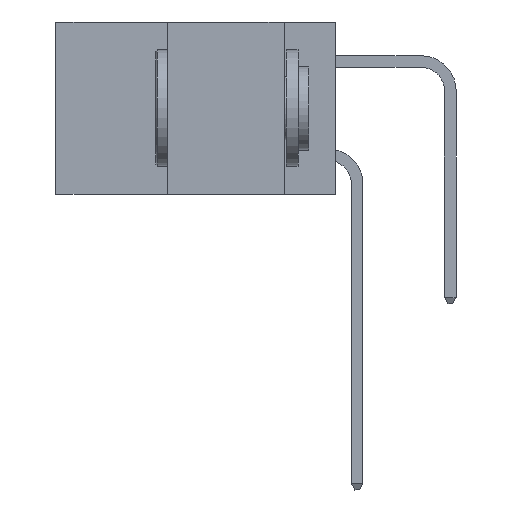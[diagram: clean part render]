
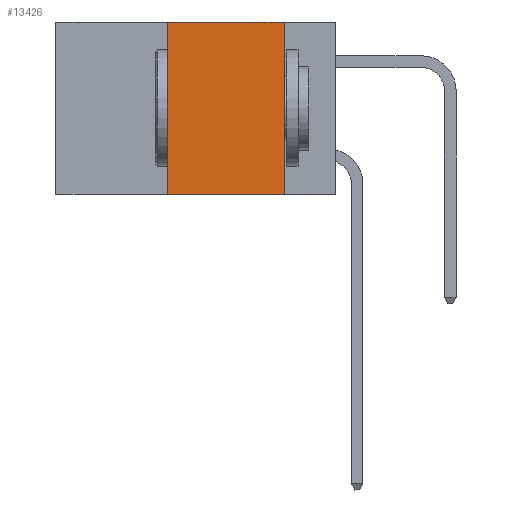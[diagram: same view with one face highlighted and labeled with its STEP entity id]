
A CAD part, left-side view. The second image highlights one B-rep face of the part: STEP entity #13426.
In plain terms, the highlighted planar face has unit normal (-1, 0, 0).
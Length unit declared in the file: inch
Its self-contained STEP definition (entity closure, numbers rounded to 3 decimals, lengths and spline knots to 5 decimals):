
#1444 = CARTESIAN_POINT ( 'NONE',  ( 0., 0.11, 0. ) ) ;
#1592 = VERTEX_POINT ( 'NONE', #6874 ) ;
#1670 = LINE ( 'NONE', #9726, #9550 ) ;
#1695 = DIRECTION ( 'NONE',  ( 0., 0., -1. ) ) ;
#2039 = LINE ( 'NONE', #3371, #7864 ) ;
#2083 = ORIENTED_EDGE ( 'NONE', *, *, #8110, .F. ) ;
#2244 = CARTESIAN_POINT ( 'NONE',  ( 0., 0.36, 0. ) ) ;
#2601 = CARTESIAN_POINT ( 'NONE',  ( 0., 0.6, 0. ) ) ;
#3084 = DIRECTION ( 'NONE',  ( 0., -1., 0. ) ) ;
#3119 = VECTOR ( 'NONE', #12470, 39.37008 ) ;
#3371 = CARTESIAN_POINT ( 'NONE',  ( 0., 0.6, -0.37 ) ) ;
#3650 = EDGE_CURVE ( 'NONE', #6396, #1592, #12769, .T. ) ;
#4830 = LINE ( 'NONE', #1444, #9013 ) ;
#4873 = DIRECTION ( 'NONE',  ( 0., 0., -1. ) ) ;
#5020 = AXIS2_PLACEMENT_3D ( 'NONE', #2601, #7124, #4873 ) ;
#5290 = EDGE_CURVE ( 'NONE', #6396, #11457, #2039, .T. ) ;
#5695 = ORIENTED_EDGE ( 'NONE', *, *, #8839, .F. ) ;
#5762 = CARTESIAN_POINT ( 'NONE',  ( 0., 0.36, -0.37 ) ) ;
#6326 = CARTESIAN_POINT ( 'NONE',  ( 0., 0.11, 0. ) ) ;
#6396 = VERTEX_POINT ( 'NONE', #5762 ) ;
#6810 = DIRECTION ( 'NONE',  ( 0., -1., 0. ) ) ;
#6874 = CARTESIAN_POINT ( 'NONE',  ( 0., 0.36, 0. ) ) ;
#6894 = ORIENTED_EDGE ( 'NONE', *, *, #3650, .F. ) ;
#7075 = PLANE ( 'NONE',  #5020 ) ;
#7124 = DIRECTION ( 'NONE',  ( 1., 0., 0. ) ) ;
#7228 = FACE_OUTER_BOUND ( 'NONE', #11441, .T. ) ;
#7864 = VECTOR ( 'NONE', #6810, 39.37008 ) ;
#8110 = EDGE_CURVE ( 'NONE', #1592, #8829, #1670, .T. ) ;
#8829 = VERTEX_POINT ( 'NONE', #6326 ) ;
#8839 = EDGE_CURVE ( 'NONE', #8829, #11457, #4830, .T. ) ;
#9013 = VECTOR ( 'NONE', #1695, 39.37008 ) ;
#9550 = VECTOR ( 'NONE', #3084, 39.37008 ) ;
#9726 = CARTESIAN_POINT ( 'NONE',  ( 0., 0.6, 0. ) ) ;
#11441 = EDGE_LOOP ( 'NONE', ( #5695, #2083, #6894, #13343 ) ) ;
#11457 = VERTEX_POINT ( 'NONE', #11888 ) ;
#11888 = CARTESIAN_POINT ( 'NONE',  ( 0., 0.11, -0.37 ) ) ;
#12470 = DIRECTION ( 'NONE',  ( 0., 0., 1. ) ) ;
#12769 = LINE ( 'NONE', #2244, #3119 ) ;
#13343 = ORIENTED_EDGE ( 'NONE', *, *, #5290, .T. ) ;
#13426 = ADVANCED_FACE ( 'NONE', ( #7228 ), #7075, .F. ) ;
